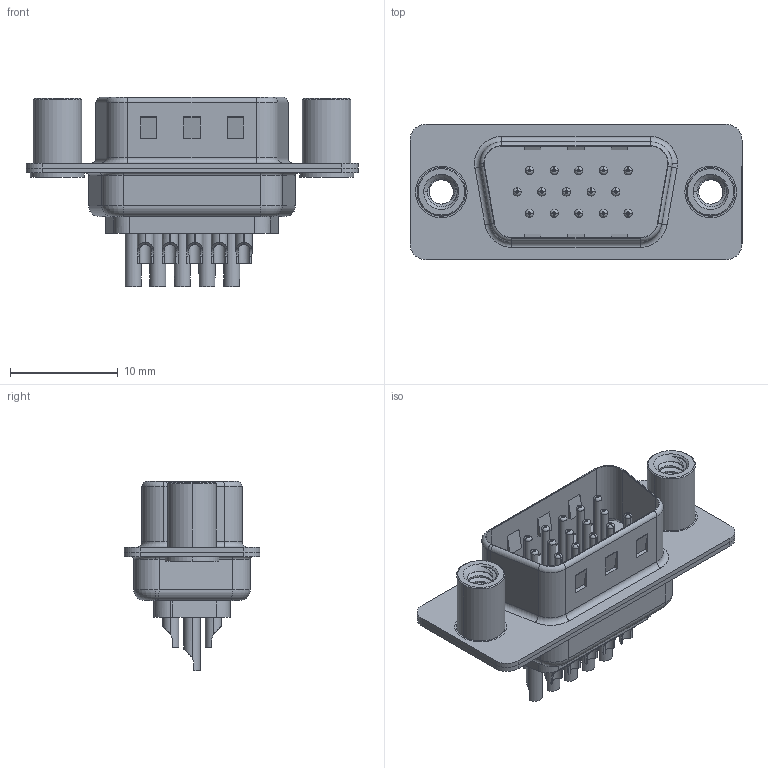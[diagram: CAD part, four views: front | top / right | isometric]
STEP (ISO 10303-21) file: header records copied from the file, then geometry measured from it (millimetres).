
FILE_DESCRIPTION (( 'STEP AP203' ), '1' );
FILE_NAME ('637-015-332-068.STEP', '2020-07-17T23:28:02', ( '' ), ( '' ), 'SwSTEP 2.0', 'SolidWorks 2020', '' );
FILE_SCHEMA (( 'CONFIG_CONTROL_DESIGN' ));
Length unit declared in the file: millimetre
Products named in the file (8): 637 4-40 Threaded Standoff; 637 Shell Rear_15 Contacts; 637 Contact Row 1_32; 637 Shell Front_15 Contacts; 637 Housing_15 Contacts; 637-015-332-068; 637 Contact Row 2_32; 637 Contact Row 3_32
Assembly tree (20 placements, depth 2):
  637-015-332-068
    637 Housing_15 Contacts
    637 Shell Front_15 Contacts
    637 Shell Rear_15 Contacts
    637 Contact Row 1_32  x5
    637 Contact Row 2_32  x5
    637 Contact Row 3_32  x5
    637 4-40 Threaded Standoff  x2
Bounding box: 30.8 x 12.6 x 17.55 mm (x, y, z)
Volume: 1393.8 mm3; surface area: 4972.1 mm2
Topology: 20 solids, 20 shells, 1298 faces, 3309 edges, 2094 vertices
Faces by surface type: cylinder 592, torus 365, plane 319, cone 16, bspline 6
Entity records: 20297 total; most frequent: CARTESIAN_POINT 4881, DIRECTION 3226, ORIENTED_EDGE 2860, EDGE_CURVE 1430, AXIS2_PLACEMENT_3D 1307, VERTEX_POINT 908, CIRCLE 711, EDGE_LOOP 672
